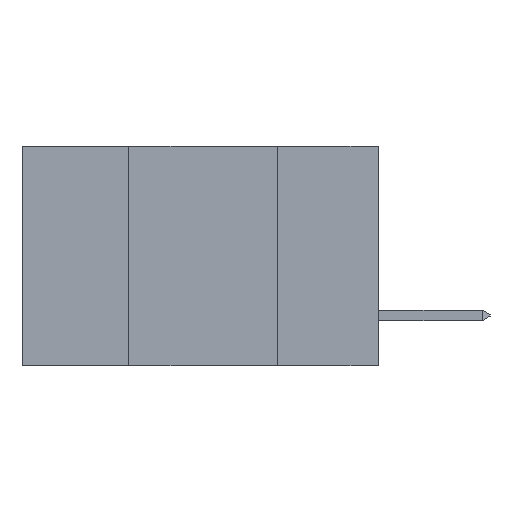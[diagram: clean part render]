
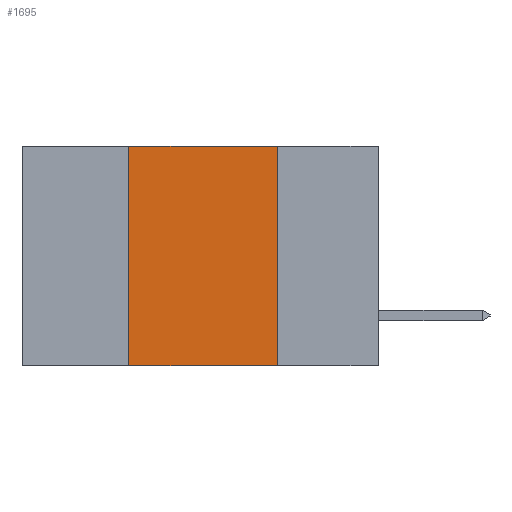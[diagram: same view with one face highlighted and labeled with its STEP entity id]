
A CAD part, left-side view. The second image highlights one B-rep face of the part: STEP entity #1695.
In plain terms, the highlighted planar face has unit normal (-1, 0, 0).
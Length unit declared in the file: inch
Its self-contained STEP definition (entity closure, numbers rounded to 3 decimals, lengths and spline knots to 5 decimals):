
#67 = VECTOR ( 'NONE', #9658, 39.37008 ) ;
#646 = VECTOR ( 'NONE', #2208, 39.37008 ) ;
#700 = PLANE ( 'NONE',  #9660 ) ;
#835 = ORIENTED_EDGE ( 'NONE', *, *, #1320, .F. ) ;
#853 = VERTEX_POINT ( 'NONE', #7210 ) ;
#1320 = EDGE_CURVE ( 'NONE', #6899, #853, #2514, .T. ) ;
#1406 = ORIENTED_EDGE ( 'NONE', *, *, #9371, .T. ) ;
#1695 = ADVANCED_FACE ( 'NONE', ( #5602 ), #700, .F. ) ;
#2208 = DIRECTION ( 'NONE',  ( 0., 0., -1. ) ) ;
#2270 = CARTESIAN_POINT ( 'NONE',  ( 0., 0.42, -0.37 ) ) ;
#2514 = LINE ( 'NONE', #6784, #67 ) ;
#2814 = LINE ( 'NONE', #7837, #646 ) ;
#2924 = EDGE_LOOP ( 'NONE', ( #7300, #6985, #835, #1406 ) ) ;
#3754 = LINE ( 'NONE', #3843, #6264 ) ;
#3843 = CARTESIAN_POINT ( 'NONE',  ( 0., 0.6, -0.37 ) ) ;
#4685 = VERTEX_POINT ( 'NONE', #6839 ) ;
#4982 = EDGE_CURVE ( 'NONE', #853, #7687, #11143, .T. ) ;
#5348 = CARTESIAN_POINT ( 'NONE',  ( 0., 0.17, 0. ) ) ;
#5407 = CARTESIAN_POINT ( 'NONE',  ( 0., 0.6, 0. ) ) ;
#5602 = FACE_OUTER_BOUND ( 'NONE', #2924, .T. ) ;
#6264 = VECTOR ( 'NONE', #10280, 39.37008 ) ;
#6784 = CARTESIAN_POINT ( 'NONE',  ( 0., 0.42, 0. ) ) ;
#6839 = CARTESIAN_POINT ( 'NONE',  ( 0., 0.17, -0.37 ) ) ;
#6899 = VERTEX_POINT ( 'NONE', #2270 ) ;
#6985 = ORIENTED_EDGE ( 'NONE', *, *, #4982, .F. ) ;
#7210 = CARTESIAN_POINT ( 'NONE',  ( 0., 0.42, 0. ) ) ;
#7300 = ORIENTED_EDGE ( 'NONE', *, *, #10183, .F. ) ;
#7687 = VERTEX_POINT ( 'NONE', #5348 ) ;
#7726 = DIRECTION ( 'NONE',  ( 0., 0., -1. ) ) ;
#7752 = DIRECTION ( 'NONE',  ( 1., 0., 0. ) ) ;
#7837 = CARTESIAN_POINT ( 'NONE',  ( 0., 0.17, 0. ) ) ;
#8219 = DIRECTION ( 'NONE',  ( 0., -1., 0. ) ) ;
#8814 = VECTOR ( 'NONE', #8219, 39.37008 ) ;
#9371 = EDGE_CURVE ( 'NONE', #6899, #4685, #3754, .T. ) ;
#9658 = DIRECTION ( 'NONE',  ( 0., 0., 1. ) ) ;
#9660 = AXIS2_PLACEMENT_3D ( 'NONE', #10488, #7752, #7726 ) ;
#10183 = EDGE_CURVE ( 'NONE', #7687, #4685, #2814, .T. ) ;
#10280 = DIRECTION ( 'NONE',  ( 0., -1., 0. ) ) ;
#10488 = CARTESIAN_POINT ( 'NONE',  ( 0., 0.6, 0. ) ) ;
#11143 = LINE ( 'NONE', #5407, #8814 ) ;
